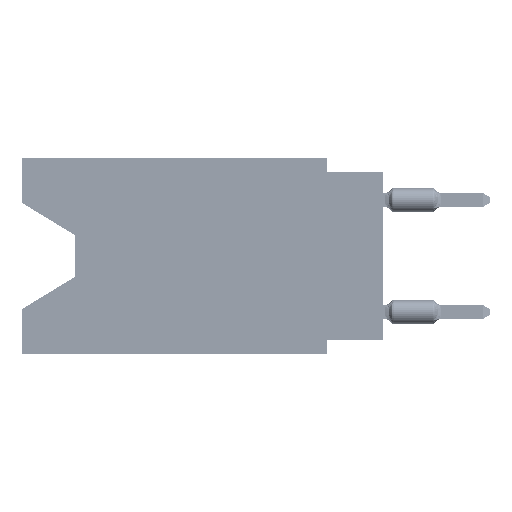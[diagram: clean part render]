
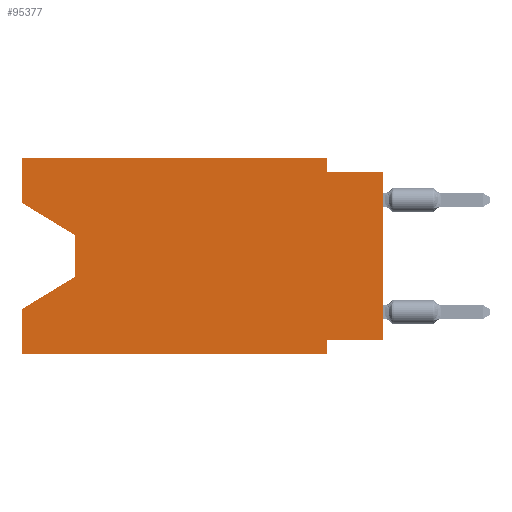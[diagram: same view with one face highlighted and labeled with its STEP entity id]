
A CAD part, left-side view. The second image highlights one B-rep face of the part: STEP entity #95377.
In plain terms, the highlighted planar face has unit normal (-1, 0, 0).
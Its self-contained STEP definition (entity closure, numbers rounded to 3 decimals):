
#3553 = VECTOR ( 'NONE', #72944, 1000. ) ;
#4962 = ORIENTED_EDGE ( 'NONE', *, *, #61805, .F. ) ;
#5272 = VECTOR ( 'NONE', #52572, 1000. ) ;
#5502 = DIRECTION ( 'NONE',  ( 0., 0., -1. ) ) ;
#6671 = DIRECTION ( 'NONE',  ( 0., 0., -1. ) ) ;
#7831 = CARTESIAN_POINT ( 'NONE',  ( 0., 16.383, -2.038 ) ) ;
#8062 = VERTEX_POINT ( 'NONE', #93461 ) ;
#8740 = EDGE_CURVE ( 'NONE', #17281, #67087, #31487, .T. ) ;
#10601 = ORIENTED_EDGE ( 'NONE', *, *, #101676, .T. ) ;
#11089 = VECTOR ( 'NONE', #75828, 1000. ) ;
#11664 = CARTESIAN_POINT ( 'NONE',  ( 0., 16.383, -8.89 ) ) ;
#13175 = DIRECTION ( 'NONE',  ( 0., -0.855, -0.519 ) ) ;
#15486 = CARTESIAN_POINT ( 'NONE',  ( 0., 2.54, -8.255 ) ) ;
#17281 = VERTEX_POINT ( 'NONE', #11664 ) ;
#17602 = VECTOR ( 'NONE', #73650, 1000. ) ;
#17950 = VECTOR ( 'NONE', #6671, 1000. ) ;
#18330 = LINE ( 'NONE', #93630, #63221 ) ;
#18562 = VECTOR ( 'NONE', #13175, 1000. ) ;
#19281 = LINE ( 'NONE', #101161, #5272 ) ;
#22396 = EDGE_CURVE ( 'NONE', #79428, #8062, #43095, .T. ) ;
#23300 = CARTESIAN_POINT ( 'NONE',  ( 0., 16.383, -8.89 ) ) ;
#24522 = LINE ( 'NONE', #57816, #17602 ) ;
#27289 = CARTESIAN_POINT ( 'NONE',  ( 0., 16.383, -6.852 ) ) ;
#28669 = EDGE_CURVE ( 'NONE', #87180, #67087, #91472, .T. ) ;
#28718 = ORIENTED_EDGE ( 'NONE', *, *, #48467, .F. ) ;
#28957 = FACE_OUTER_BOUND ( 'NONE', #30909, .T. ) ;
#30909 = EDGE_LOOP ( 'NONE', ( #10601, #73337, #57655, #60908, #98486, #40122, #28718, #38624, #4962, #31865, #79337, #98908 ) ) ;
#31487 = LINE ( 'NONE', #23300, #68262 ) ;
#31809 = VERTEX_POINT ( 'NONE', #34517 ) ;
#31865 = ORIENTED_EDGE ( 'NONE', *, *, #62728, .F. ) ;
#33208 = LINE ( 'NONE', #66492, #50833 ) ;
#33471 = LINE ( 'NONE', #68347, #47459 ) ;
#34517 = CARTESIAN_POINT ( 'NONE',  ( 0., 13.97, -3.505 ) ) ;
#37155 = CARTESIAN_POINT ( 'NONE',  ( 0., 16.383, 0. ) ) ;
#37698 = PLANE ( 'NONE',  #56019 ) ;
#38624 = ORIENTED_EDGE ( 'NONE', *, *, #22396, .T. ) ;
#39125 = CARTESIAN_POINT ( 'NONE',  ( 0., 2.54, -8.89 ) ) ;
#40122 = ORIENTED_EDGE ( 'NONE', *, *, #28669, .F. ) ;
#41509 = CARTESIAN_POINT ( 'NONE',  ( 0., 16.383, 0. ) ) ;
#41956 = LINE ( 'NONE', #44109, #82121 ) ;
#43095 = LINE ( 'NONE', #68733, #11089 ) ;
#44109 = CARTESIAN_POINT ( 'NONE',  ( 0., 13.97, -3.505 ) ) ;
#45748 = VERTEX_POINT ( 'NONE', #27289 ) ;
#47459 = VECTOR ( 'NONE', #83612, 1000. ) ;
#48467 = EDGE_CURVE ( 'NONE', #79428, #87180, #33208, .T. ) ;
#50833 = VECTOR ( 'NONE', #74135, 1000. ) ;
#52572 = DIRECTION ( 'NONE',  ( 0., -1., 0. ) ) ;
#53744 = VERTEX_POINT ( 'NONE', #92317 ) ;
#55123 = DIRECTION ( 'NONE',  ( 1., 0., 0. ) ) ;
#56019 = AXIS2_PLACEMENT_3D ( 'NONE', #37155, #55123, #5502 ) ;
#56300 = CARTESIAN_POINT ( 'NONE',  ( 0., 0., -8.255 ) ) ;
#56535 = CARTESIAN_POINT ( 'NONE',  ( 0., 2.54, 0. ) ) ;
#56580 = DIRECTION ( 'NONE',  ( 0., -1., 0. ) ) ;
#57655 = ORIENTED_EDGE ( 'NONE', *, *, #85995, .T. ) ;
#57816 = CARTESIAN_POINT ( 'NONE',  ( 0., 16.383, 0. ) ) ;
#58744 = DIRECTION ( 'NONE',  ( 0., -1., 0. ) ) ;
#58870 = VERTEX_POINT ( 'NONE', #82253 ) ;
#59426 = EDGE_CURVE ( 'NONE', #53744, #104820, #19281, .T. ) ;
#60908 = ORIENTED_EDGE ( 'NONE', *, *, #66351, .F. ) ;
#61805 = EDGE_CURVE ( 'NONE', #58870, #8062, #18330, .T. ) ;
#62728 = EDGE_CURVE ( 'NONE', #104820, #58870, #97785, .T. ) ;
#63221 = VECTOR ( 'NONE', #58744, 1000. ) ;
#64457 = CARTESIAN_POINT ( 'NONE',  ( 0., 16.383, -2.038 ) ) ;
#66351 = EDGE_CURVE ( 'NONE', #17281, #45748, #90077, .T. ) ;
#66492 = CARTESIAN_POINT ( 'NONE',  ( 0., 0., -8.255 ) ) ;
#66884 = VERTEX_POINT ( 'NONE', #85485 ) ;
#67087 = VERTEX_POINT ( 'NONE', #88732 ) ;
#68262 = VECTOR ( 'NONE', #56580, 1000. ) ;
#68347 = CARTESIAN_POINT ( 'NONE',  ( 0., 13.97, -5.385 ) ) ;
#68733 = CARTESIAN_POINT ( 'NONE',  ( 0., 0., 0. ) ) ;
#72944 = DIRECTION ( 'NONE',  ( 0., 0., -1. ) ) ;
#73337 = ORIENTED_EDGE ( 'NONE', *, *, #93267, .T. ) ;
#73650 = DIRECTION ( 'NONE',  ( 0., 0., 1. ) ) ;
#74135 = DIRECTION ( 'NONE',  ( 0., 1., 0. ) ) ;
#74774 = DIRECTION ( 'NONE',  ( 0., 0., 1. ) ) ;
#75828 = DIRECTION ( 'NONE',  ( 0., 0., 1. ) ) ;
#76845 = DIRECTION ( 'NONE',  ( 0., 0., -1. ) ) ;
#79203 = LINE ( 'NONE', #64457, #18562 ) ;
#79337 = ORIENTED_EDGE ( 'NONE', *, *, #59426, .F. ) ;
#79428 = VERTEX_POINT ( 'NONE', #56300 ) ;
#82121 = VECTOR ( 'NONE', #76845, 1000. ) ;
#82253 = CARTESIAN_POINT ( 'NONE',  ( 0., 2.54, -0.635 ) ) ;
#83575 = VERTEX_POINT ( 'NONE', #7831 ) ;
#83612 = DIRECTION ( 'NONE',  ( 0., 0.855, -0.519 ) ) ;
#85485 = CARTESIAN_POINT ( 'NONE',  ( 0., 13.97, -5.385 ) ) ;
#85995 = EDGE_CURVE ( 'NONE', #66884, #45748, #33471, .T. ) ;
#87180 = VERTEX_POINT ( 'NONE', #15486 ) ;
#88732 = CARTESIAN_POINT ( 'NONE',  ( 0., 2.54, -8.89 ) ) ;
#89599 = CARTESIAN_POINT ( 'NONE',  ( 0., 2.54, 0. ) ) ;
#90077 = LINE ( 'NONE', #41509, #106621 ) ;
#91472 = LINE ( 'NONE', #39125, #3553 ) ;
#92317 = CARTESIAN_POINT ( 'NONE',  ( 0., 16.383, 0. ) ) ;
#93040 = EDGE_CURVE ( 'NONE', #83575, #53744, #24522, .T. ) ;
#93267 = EDGE_CURVE ( 'NONE', #31809, #66884, #41956, .T. ) ;
#93461 = CARTESIAN_POINT ( 'NONE',  ( 0., 0., -0.635 ) ) ;
#93630 = CARTESIAN_POINT ( 'NONE',  ( 0., 0., -0.635 ) ) ;
#95377 = ADVANCED_FACE ( 'NONE', ( #28957 ), #37698, .F. ) ;
#97785 = LINE ( 'NONE', #89599, #17950 ) ;
#98486 = ORIENTED_EDGE ( 'NONE', *, *, #8740, .T. ) ;
#98908 = ORIENTED_EDGE ( 'NONE', *, *, #93040, .F. ) ;
#101161 = CARTESIAN_POINT ( 'NONE',  ( 0., 16.383, 0. ) ) ;
#101676 = EDGE_CURVE ( 'NONE', #83575, #31809, #79203, .T. ) ;
#104820 = VERTEX_POINT ( 'NONE', #56535 ) ;
#106621 = VECTOR ( 'NONE', #74774, 1000. ) ;
